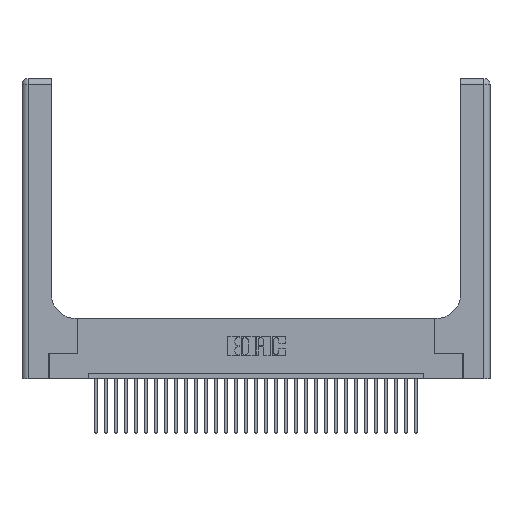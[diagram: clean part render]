
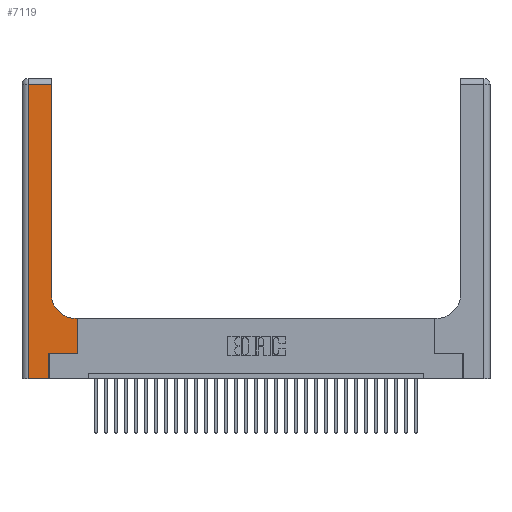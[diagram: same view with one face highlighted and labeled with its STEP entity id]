
A CAD part, top view. The second image highlights one B-rep face of the part: STEP entity #7119.
In plain terms, the highlighted planar face has unit normal (0, 0, 1).
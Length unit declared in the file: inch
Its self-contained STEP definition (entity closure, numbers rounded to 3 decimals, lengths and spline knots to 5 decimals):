
#32 = VERTEX_POINT ( 'NONE', #29745 ) ;
#1581 = CARTESIAN_POINT ( 'NONE',  ( 0., 2.94, 0.37 ) ) ;
#1740 = DIRECTION ( 'NONE',  ( 0., 1., 0. ) ) ;
#1917 = ORIENTED_EDGE ( 'NONE', *, *, #8241, .T. ) ;
#2361 = VECTOR ( 'NONE', #20776, 39.37008 ) ;
#2738 = DIRECTION ( 'NONE',  ( -1., 0., 0. ) ) ;
#3092 = ORIENTED_EDGE ( 'NONE', *, *, #16967, .T. ) ;
#3254 = VECTOR ( 'NONE', #19660, 39.37008 ) ;
#3509 = ORIENTED_EDGE ( 'NONE', *, *, #7537, .T. ) ;
#4108 = EDGE_CURVE ( 'NONE', #14741, #26675, #28138, .T. ) ;
#4445 = CARTESIAN_POINT ( 'NONE',  ( 0., 0., 0.37 ) ) ;
#4772 = DIRECTION ( 'NONE',  ( 0., 1., 0. ) ) ;
#5346 = CARTESIAN_POINT ( 'NONE',  ( 0.5415, 0.85, 0.37 ) ) ;
#5563 = VECTOR ( 'NONE', #22674, 39.37008 ) ;
#5583 = DIRECTION ( 'NONE',  ( -1., 0., 0. ) ) ;
#7119 = ADVANCED_FACE ( 'NONE', ( #20449 ), #17615, .F. ) ;
#7288 = AXIS2_PLACEMENT_3D ( 'NONE', #29735, #10561, #5583 ) ;
#7537 = EDGE_CURVE ( 'NONE', #11683, #29596, #10250, .T. ) ;
#7980 = LINE ( 'NONE', #1581, #2361 ) ;
#8241 = EDGE_CURVE ( 'NONE', #32, #27157, #16636, .T. ) ;
#9124 = CARTESIAN_POINT ( 'NONE',  ( 0.269, 0., 0.37 ) ) ;
#9630 = CARTESIAN_POINT ( 'NONE',  ( 0.2915, 2.94, 0.37 ) ) ;
#10246 = CARTESIAN_POINT ( 'NONE',  ( 0.06, 3., 0.37 ) ) ;
#10250 = LINE ( 'NONE', #15896, #18557 ) ;
#10526 = ORIENTED_EDGE ( 'NONE', *, *, #29343, .T. ) ;
#10561 = DIRECTION ( 'NONE',  ( 0., 0., -1. ) ) ;
#11047 = LINE ( 'NONE', #9124, #29501 ) ;
#11256 = LINE ( 'NONE', #13323, #5563 ) ;
#11683 = VERTEX_POINT ( 'NONE', #23811 ) ;
#11735 = DIRECTION ( 'NONE',  ( 1., 0., 0. ) ) ;
#11851 = ORIENTED_EDGE ( 'NONE', *, *, #15916, .T. ) ;
#12514 = VERTEX_POINT ( 'NONE', #30798 ) ;
#12848 = DIRECTION ( 'NONE',  ( 0., 0., -1. ) ) ;
#13323 = CARTESIAN_POINT ( 'NONE',  ( 0.2915, 3., 0.37 ) ) ;
#13643 = EDGE_CURVE ( 'NONE', #27792, #14741, #7980, .T. ) ;
#14741 = VERTEX_POINT ( 'NONE', #24099 ) ;
#15799 = AXIS2_PLACEMENT_3D ( 'NONE', #5346, #12848, #27492 ) ;
#15896 = CARTESIAN_POINT ( 'NONE',  ( 0.269, 0.25, 0.37 ) ) ;
#15916 = EDGE_CURVE ( 'NONE', #12514, #27792, #11256, .T. ) ;
#16636 = LINE ( 'NONE', #17177, #20388 ) ;
#16715 = CARTESIAN_POINT ( 'NONE',  ( 0.5585, 0.25, 0.37 ) ) ;
#16967 = EDGE_CURVE ( 'NONE', #26675, #17671, #27484, .T. ) ;
#17177 = CARTESIAN_POINT ( 'NONE',  ( 0.2915, 0.6, 0.37 ) ) ;
#17615 = PLANE ( 'NONE',  #7288 ) ;
#17671 = VERTEX_POINT ( 'NONE', #29164 ) ;
#18557 = VECTOR ( 'NONE', #20918, 39.37008 ) ;
#18852 = EDGE_CURVE ( 'NONE', #29596, #32, #30020, .T. ) ;
#19660 = DIRECTION ( 'NONE',  ( 0., -1., 0. ) ) ;
#20388 = VECTOR ( 'NONE', #2738, 39.37008 ) ;
#20449 = FACE_OUTER_BOUND ( 'NONE', #21424, .T. ) ;
#20721 = CARTESIAN_POINT ( 'NONE',  ( 0.06, 0., 0.37 ) ) ;
#20776 = DIRECTION ( 'NONE',  ( -1., 0., 0. ) ) ;
#20918 = DIRECTION ( 'NONE',  ( 1., 0., 0. ) ) ;
#21424 = EDGE_LOOP ( 'NONE', ( #11851, #24051, #29948, #3092, #10526, #3509, #25597, #1917, #27555 ) ) ;
#22674 = DIRECTION ( 'NONE',  ( 0., 1., 0. ) ) ;
#23811 = CARTESIAN_POINT ( 'NONE',  ( 0.269, 0.25, 0.37 ) ) ;
#24051 = ORIENTED_EDGE ( 'NONE', *, *, #13643, .T. ) ;
#24099 = CARTESIAN_POINT ( 'NONE',  ( 0.06, 2.94, 0.37 ) ) ;
#25597 = ORIENTED_EDGE ( 'NONE', *, *, #18852, .T. ) ;
#25878 = CIRCLE ( 'NONE', #15799, 0.25 ) ;
#26675 = VERTEX_POINT ( 'NONE', #20721 ) ;
#26720 = VECTOR ( 'NONE', #11735, 39.37008 ) ;
#27000 = VECTOR ( 'NONE', #4772, 39.37008 ) ;
#27099 = EDGE_CURVE ( 'NONE', #27157, #12514, #25878, .T. ) ;
#27157 = VERTEX_POINT ( 'NONE', #29488 ) ;
#27484 = LINE ( 'NONE', #4445, #26720 ) ;
#27492 = DIRECTION ( 'NONE',  ( 1., 0., 0. ) ) ;
#27555 = ORIENTED_EDGE ( 'NONE', *, *, #27099, .T. ) ;
#27792 = VERTEX_POINT ( 'NONE', #9630 ) ;
#28138 = LINE ( 'NONE', #10246, #3254 ) ;
#29164 = CARTESIAN_POINT ( 'NONE',  ( 0.269, 0., 0.37 ) ) ;
#29324 = CARTESIAN_POINT ( 'NONE',  ( 0.5585, 0.25, 0.37 ) ) ;
#29343 = EDGE_CURVE ( 'NONE', #17671, #11683, #11047, .T. ) ;
#29488 = CARTESIAN_POINT ( 'NONE',  ( 0.5415, 0.6, 0.37 ) ) ;
#29501 = VECTOR ( 'NONE', #1740, 39.37008 ) ;
#29596 = VERTEX_POINT ( 'NONE', #29324 ) ;
#29735 = CARTESIAN_POINT ( 'NONE',  ( 0., 3., 0.37 ) ) ;
#29745 = CARTESIAN_POINT ( 'NONE',  ( 0.5585, 0.6, 0.37 ) ) ;
#29948 = ORIENTED_EDGE ( 'NONE', *, *, #4108, .T. ) ;
#30020 = LINE ( 'NONE', #16715, #27000 ) ;
#30798 = CARTESIAN_POINT ( 'NONE',  ( 0.2915, 0.85, 0.37 ) ) ;
